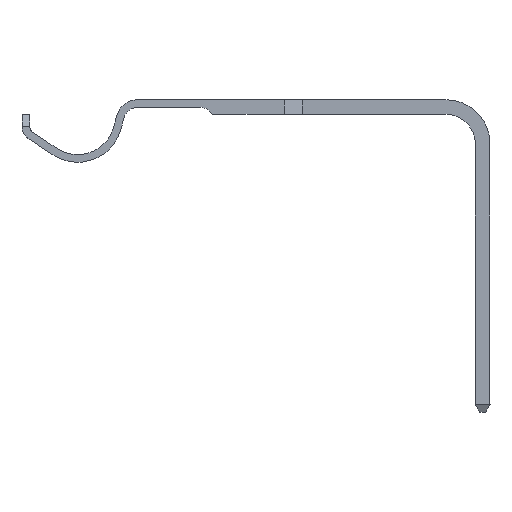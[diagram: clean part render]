
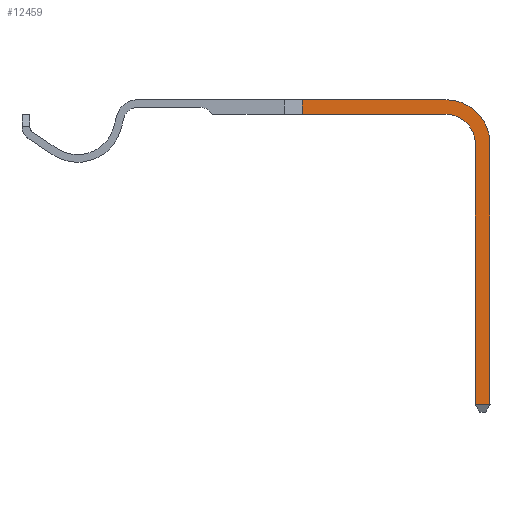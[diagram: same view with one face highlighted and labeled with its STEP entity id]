
A CAD part, left-side view. The second image highlights one B-rep face of the part: STEP entity #12459.
In plain terms, the highlighted face is planar.
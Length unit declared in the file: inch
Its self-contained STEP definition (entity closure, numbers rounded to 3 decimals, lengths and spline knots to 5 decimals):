
#780 = DIRECTION ( 'NONE',  ( 1., 0., 0. ) ) ;
#1113 = CARTESIAN_POINT ( 'NONE',  ( 0.61115, 0.0375, -0.0125 ) ) ;
#1252 = CARTESIAN_POINT ( 'NONE',  ( 0.90571, 0.532, -0.0125 ) ) ;
#1260 = CIRCLE ( 'NONE', #6583, 0.05 ) ;
#1433 = DIRECTION ( 'NONE',  ( 1., 0., 0. ) ) ;
#1563 = CARTESIAN_POINT ( 'NONE',  ( 0.93071, 0.532, -0.0125 ) ) ;
#2272 = ORIENTED_EDGE ( 'NONE', *, *, #16810, .T. ) ;
#2661 = CARTESIAN_POINT ( 'NONE',  ( 0.85571, 0.0125, -0.0125 ) ) ;
#3367 = EDGE_LOOP ( 'NONE', ( #12731, #2272, #11298, #8935, #4528, #12847, #11060, #4565 ) ) ;
#3960 = CARTESIAN_POINT ( 'NONE',  ( 0.93071, 0.0875, -0.0125 ) ) ;
#4528 = ORIENTED_EDGE ( 'NONE', *, *, #6221, .T. ) ;
#4565 = ORIENTED_EDGE ( 'NONE', *, *, #6524, .T. ) ;
#5339 = VERTEX_POINT ( 'NONE', #1563 ) ;
#5464 = DIRECTION ( 'NONE',  ( 0., 0., -1. ) ) ;
#5566 = LINE ( 'NONE', #17778, #13659 ) ;
#5818 = AXIS2_PLACEMENT_3D ( 'NONE', #8533, #19863, #10163 ) ;
#6221 = EDGE_CURVE ( 'NONE', #18647, #19989, #15008, .T. ) ;
#6281 = DIRECTION ( 'NONE',  ( 1., 0., 0. ) ) ;
#6488 = CARTESIAN_POINT ( 'NONE',  ( 0.85571, 0.0375, -0.0125 ) ) ;
#6524 = EDGE_CURVE ( 'NONE', #15290, #7083, #1260, .T. ) ;
#6583 = AXIS2_PLACEMENT_3D ( 'NONE', #20853, #11201, #1433 ) ;
#6812 = VECTOR ( 'NONE', #780, 39.37008 ) ;
#7083 = VERTEX_POINT ( 'NONE', #7713 ) ;
#7166 = CARTESIAN_POINT ( 'NONE',  ( 0.58021, 0.0125, -0.0125 ) ) ;
#7236 = VECTOR ( 'NONE', #9205, 39.37008 ) ;
#7565 = CARTESIAN_POINT ( 'NONE',  ( 0.61115, 0.0875, -0.0125 ) ) ;
#7624 = AXIS2_PLACEMENT_3D ( 'NONE', #15179, #5464, #16802 ) ;
#7649 = VECTOR ( 'NONE', #16863, 39.37008 ) ;
#7713 = CARTESIAN_POINT ( 'NONE',  ( 0.90571, 0.0875, -0.0125 ) ) ;
#7901 = CARTESIAN_POINT ( 'NONE',  ( 0.93071, 0.0875, -0.0125 ) ) ;
#8416 = CARTESIAN_POINT ( 'NONE',  ( 0.61115, 0.0125, -0.0125 ) ) ;
#8533 = CARTESIAN_POINT ( 'NONE',  ( 0.85571, 0.0875, -0.0125 ) ) ;
#8935 = ORIENTED_EDGE ( 'NONE', *, *, #15537, .T. ) ;
#8975 = EDGE_CURVE ( 'NONE', #19989, #15101, #15846, .T. ) ;
#9205 = DIRECTION ( 'NONE',  ( 0., 1., 0. ) ) ;
#9751 = VERTEX_POINT ( 'NONE', #7901 ) ;
#10095 = PLANE ( 'NONE',  #5818 ) ;
#10163 = DIRECTION ( 'NONE',  ( 1., 0., 0. ) ) ;
#10247 = VERTEX_POINT ( 'NONE', #1252 ) ;
#10709 = VECTOR ( 'NONE', #20120, 39.37008 ) ;
#10710 = EDGE_CURVE ( 'NONE', #5339, #9751, #20551, .T. ) ;
#10877 = FACE_OUTER_BOUND ( 'NONE', #3367, .T. ) ;
#11060 = ORIENTED_EDGE ( 'NONE', *, *, #18535, .T. ) ;
#11127 = LINE ( 'NONE', #20228, #6812 ) ;
#11201 = DIRECTION ( 'NONE',  ( 0., 0., 1. ) ) ;
#11298 = ORIENTED_EDGE ( 'NONE', *, *, #10710, .T. ) ;
#12459 = ADVANCED_FACE ( 'NONE', ( #10877 ), #10095, .F. ) ;
#12731 = ORIENTED_EDGE ( 'NONE', *, *, #16875, .T. ) ;
#12847 = ORIENTED_EDGE ( 'NONE', *, *, #8975, .T. ) ;
#13659 = VECTOR ( 'NONE', #14504, 39.37008 ) ;
#14504 = DIRECTION ( 'NONE',  ( 0., 1., 0. ) ) ;
#14711 = VECTOR ( 'NONE', #6281, 39.37008 ) ;
#15008 = LINE ( 'NONE', #7166, #10709 ) ;
#15101 = VERTEX_POINT ( 'NONE', #1113 ) ;
#15179 = CARTESIAN_POINT ( 'NONE',  ( 0.85571, 0.0875, -0.0125 ) ) ;
#15207 = LINE ( 'NONE', #17636, #14711 ) ;
#15290 = VERTEX_POINT ( 'NONE', #6488 ) ;
#15537 = EDGE_CURVE ( 'NONE', #9751, #18647, #19601, .T. ) ;
#15846 = LINE ( 'NONE', #7565, #7236 ) ;
#16802 = DIRECTION ( 'NONE',  ( 1., 0., 0. ) ) ;
#16810 = EDGE_CURVE ( 'NONE', #10247, #5339, #15207, .T. ) ;
#16863 = DIRECTION ( 'NONE',  ( 0., -1., 0. ) ) ;
#16875 = EDGE_CURVE ( 'NONE', #7083, #10247, #5566, .T. ) ;
#17636 = CARTESIAN_POINT ( 'NONE',  ( 0.85571, 0.532, -0.0125 ) ) ;
#17778 = CARTESIAN_POINT ( 'NONE',  ( 0.90571, 0.0875, -0.0125 ) ) ;
#18535 = EDGE_CURVE ( 'NONE', #15101, #15290, #11127, .T. ) ;
#18647 = VERTEX_POINT ( 'NONE', #2661 ) ;
#19601 = CIRCLE ( 'NONE', #7624, 0.075 ) ;
#19863 = DIRECTION ( 'NONE',  ( 0., 0., 1. ) ) ;
#19989 = VERTEX_POINT ( 'NONE', #8416 ) ;
#20120 = DIRECTION ( 'NONE',  ( -1., 0., 0. ) ) ;
#20228 = CARTESIAN_POINT ( 'NONE',  ( 0.58021, 0.0375, -0.0125 ) ) ;
#20551 = LINE ( 'NONE', #3960, #7649 ) ;
#20853 = CARTESIAN_POINT ( 'NONE',  ( 0.85571, 0.0875, -0.0125 ) ) ;
